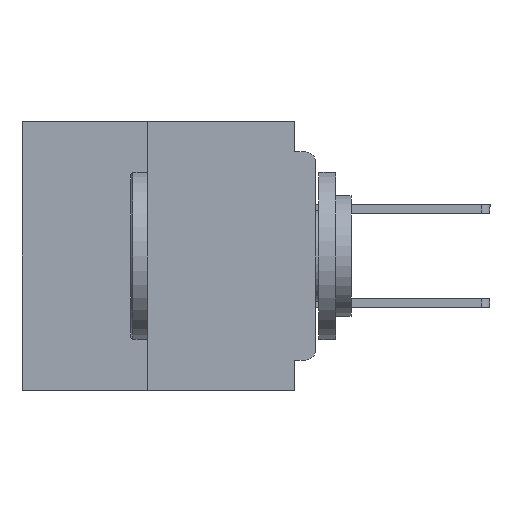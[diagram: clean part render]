
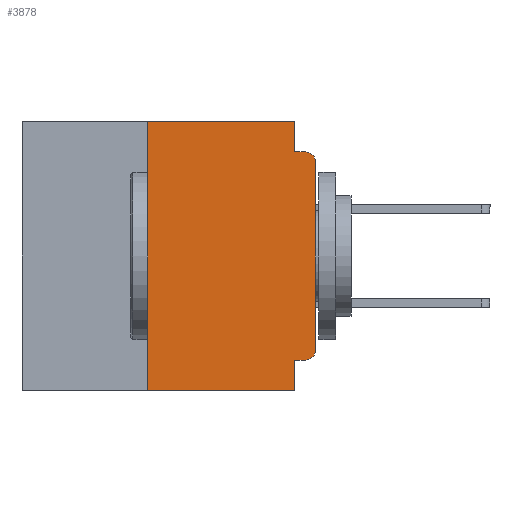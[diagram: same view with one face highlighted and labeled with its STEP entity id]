
A CAD part, left-side view. The second image highlights one B-rep face of the part: STEP entity #3878.
In plain terms, the highlighted planar face has unit normal (-1, 0, 0).
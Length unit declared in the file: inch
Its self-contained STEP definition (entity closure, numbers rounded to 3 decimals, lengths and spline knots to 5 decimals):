
#1227 = LINE ( 'NONE', #20251, #41734 ) ;
#1323 = EDGE_CURVE ( 'NONE', #47325, #48021, #35878, .T. ) ;
#2443 = ORIENTED_EDGE ( 'NONE', *, *, #41332, .F. ) ;
#2744 = CARTESIAN_POINT ( 'NONE',  ( 0., 0.031, -0.4 ) ) ;
#2831 = VERTEX_POINT ( 'NONE', #16619 ) ;
#3878 = ADVANCED_FACE ( 'NONE', ( #11738 ), #40988, .F. ) ;
#4391 = CARTESIAN_POINT ( 'NONE',  ( 0., 0.437, -0.4 ) ) ;
#4549 = VERTEX_POINT ( 'NONE', #34776 ) ;
#6155 = AXIS2_PLACEMENT_3D ( 'NONE', #43136, #19771, #47063 ) ;
#7638 = EDGE_CURVE ( 'NONE', #41064, #15888, #49956, .T. ) ;
#8456 = VECTOR ( 'NONE', #23630, 39.37008 ) ;
#8559 = ORIENTED_EDGE ( 'NONE', *, *, #43374, .T. ) ;
#8642 = EDGE_CURVE ( 'NONE', #28093, #35751, #32788, .T. ) ;
#9271 = CARTESIAN_POINT ( 'NONE',  ( 0., 0.031, -0.045 ) ) ;
#9333 = VERTEX_POINT ( 'NONE', #2744 ) ;
#9672 = CARTESIAN_POINT ( 'NONE',  ( 0., 0.25, -0.4 ) ) ;
#10453 = CARTESIAN_POINT ( 'NONE',  ( 0., 0., -0.34 ) ) ;
#11120 = VECTOR ( 'NONE', #35758, 39.37008 ) ;
#11738 = FACE_OUTER_BOUND ( 'NONE', #44143, .T. ) ;
#11854 = AXIS2_PLACEMENT_3D ( 'NONE', #38683, #38500, #38457 ) ;
#12949 = AXIS2_PLACEMENT_3D ( 'NONE', #44087, #20751, #48051 ) ;
#15096 = VECTOR ( 'NONE', #47987, 39.37008 ) ;
#15529 = ORIENTED_EDGE ( 'NONE', *, *, #16259, .F. ) ;
#15888 = VERTEX_POINT ( 'NONE', #25718 ) ;
#15950 = CIRCLE ( 'NONE', #6155, 0.015 ) ;
#16060 = ORIENTED_EDGE ( 'NONE', *, *, #8642, .T. ) ;
#16259 = EDGE_CURVE ( 'NONE', #4549, #2831, #1227, .T. ) ;
#16619 = CARTESIAN_POINT ( 'NONE',  ( 0., 0.031, 0. ) ) ;
#17809 = LINE ( 'NONE', #42449, #48981 ) ;
#18505 = EDGE_CURVE ( 'NONE', #38653, #9333, #31900, .T. ) ;
#18795 = VECTOR ( 'NONE', #33878, 39.37008 ) ;
#19273 = ORIENTED_EDGE ( 'NONE', *, *, #7638, .F. ) ;
#19379 = CARTESIAN_POINT ( 'NONE',  ( 0., 0.031, -0.4 ) ) ;
#19771 = DIRECTION ( 'NONE',  ( -1., 0., 0. ) ) ;
#20251 = CARTESIAN_POINT ( 'NONE',  ( 0., 0.437, 0. ) ) ;
#20751 = DIRECTION ( 'NONE',  ( -1., 0., 0. ) ) ;
#23630 = DIRECTION ( 'NONE',  ( 0., 0., 1. ) ) ;
#23665 = VECTOR ( 'NONE', #45663, 39.37008 ) ;
#23877 = ORIENTED_EDGE ( 'NONE', *, *, #31575, .F. ) ;
#25718 = CARTESIAN_POINT ( 'NONE',  ( 0., 0.015, -0.045 ) ) ;
#25720 = ORIENTED_EDGE ( 'NONE', *, *, #1323, .F. ) ;
#27386 = ORIENTED_EDGE ( 'NONE', *, *, #50197, .F. ) ;
#27450 = CARTESIAN_POINT ( 'NONE',  ( 0., 0., -0.045 ) ) ;
#27668 = EDGE_CURVE ( 'NONE', #35751, #15888, #15950, .T. ) ;
#28093 = VERTEX_POINT ( 'NONE', #10453 ) ;
#29214 = CARTESIAN_POINT ( 'NONE',  ( 0., 0.015, -0.355 ) ) ;
#29976 = CARTESIAN_POINT ( 'NONE',  ( 0., 0.031, -0.355 ) ) ;
#30098 = CARTESIAN_POINT ( 'NONE',  ( 0., 0., 0. ) ) ;
#30689 = ORIENTED_EDGE ( 'NONE', *, *, #18505, .T. ) ;
#31575 = EDGE_CURVE ( 'NONE', #38653, #4549, #39704, .T. ) ;
#31900 = LINE ( 'NONE', #4391, #11120 ) ;
#32712 = CIRCLE ( 'NONE', #12949, 0.015 ) ;
#32788 = LINE ( 'NONE', #30098, #23665 ) ;
#33878 = DIRECTION ( 'NONE',  ( 0., -1., 0. ) ) ;
#33905 = ORIENTED_EDGE ( 'NONE', *, *, #27668, .T. ) ;
#34596 = DIRECTION ( 'NONE',  ( 0., 0., -1. ) ) ;
#34776 = CARTESIAN_POINT ( 'NONE',  ( 0., 0.25, 0. ) ) ;
#35478 = LINE ( 'NONE', #19379, #43412 ) ;
#35751 = VERTEX_POINT ( 'NONE', #38731 ) ;
#35758 = DIRECTION ( 'NONE',  ( 0., -1., 0. ) ) ;
#35878 = LINE ( 'NONE', #46769, #15096 ) ;
#35927 = DIRECTION ( 'NONE',  ( 0., -1., 0. ) ) ;
#38457 = DIRECTION ( 'NONE',  ( 0., 0., -1. ) ) ;
#38500 = DIRECTION ( 'NONE',  ( 1., 0., 0. ) ) ;
#38653 = VERTEX_POINT ( 'NONE', #9672 ) ;
#38683 = CARTESIAN_POINT ( 'NONE',  ( 0., 0.437, 0. ) ) ;
#38731 = CARTESIAN_POINT ( 'NONE',  ( 0., 0., -0.06 ) ) ;
#39704 = LINE ( 'NONE', #43064, #8456 ) ;
#40988 = PLANE ( 'NONE',  #11854 ) ;
#41064 = VERTEX_POINT ( 'NONE', #9271 ) ;
#41332 = EDGE_CURVE ( 'NONE', #48021, #9333, #35478, .T. ) ;
#41734 = VECTOR ( 'NONE', #35927, 39.37008 ) ;
#42449 = CARTESIAN_POINT ( 'NONE',  ( 0., 0.031, 0. ) ) ;
#42741 = DIRECTION ( 'NONE',  ( 0., 0., -1. ) ) ;
#43064 = CARTESIAN_POINT ( 'NONE',  ( 0., 0.25, -0.4 ) ) ;
#43136 = CARTESIAN_POINT ( 'NONE',  ( 0., 0.015, -0.06 ) ) ;
#43374 = EDGE_CURVE ( 'NONE', #47325, #28093, #32712, .T. ) ;
#43412 = VECTOR ( 'NONE', #42741, 39.37008 ) ;
#44087 = CARTESIAN_POINT ( 'NONE',  ( 0., 0.015, -0.34 ) ) ;
#44143 = EDGE_LOOP ( 'NONE', ( #16060, #33905, #19273, #27386, #15529, #23877, #30689, #2443, #25720, #8559 ) ) ;
#45663 = DIRECTION ( 'NONE',  ( 0., 0., 1. ) ) ;
#46769 = CARTESIAN_POINT ( 'NONE',  ( 0., 0., -0.355 ) ) ;
#47063 = DIRECTION ( 'NONE',  ( 0., 0., -1. ) ) ;
#47325 = VERTEX_POINT ( 'NONE', #29214 ) ;
#47987 = DIRECTION ( 'NONE',  ( 0., 1., 0. ) ) ;
#48021 = VERTEX_POINT ( 'NONE', #29976 ) ;
#48051 = DIRECTION ( 'NONE',  ( 0., 0., -1. ) ) ;
#48981 = VECTOR ( 'NONE', #34596, 39.37008 ) ;
#49956 = LINE ( 'NONE', #27450, #18795 ) ;
#50197 = EDGE_CURVE ( 'NONE', #2831, #41064, #17809, .T. ) ;
